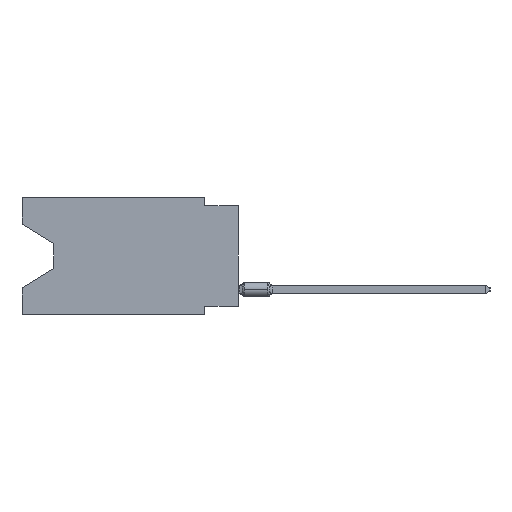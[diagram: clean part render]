
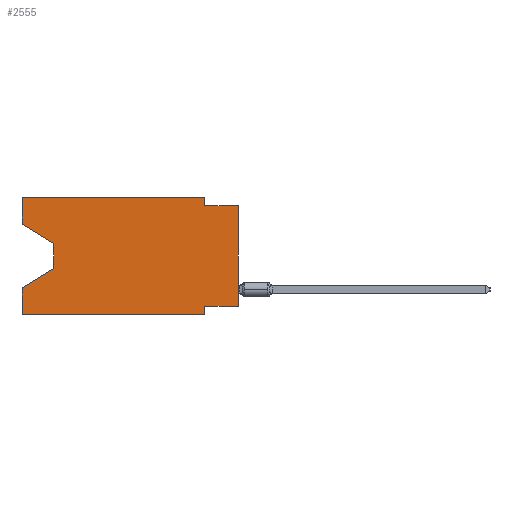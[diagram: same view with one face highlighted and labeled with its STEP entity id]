
A CAD part, left-side view. The second image highlights one B-rep face of the part: STEP entity #2555.
In plain terms, the highlighted planar face has unit normal (-1, 0, 0).
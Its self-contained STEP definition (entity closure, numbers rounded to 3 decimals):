
#773 = CARTESIAN_POINT ( 'NONE',  ( 0., 0., -8.255 ) ) ;
#1943 = VERTEX_POINT ( 'NONE', #59058 ) ;
#2044 = DIRECTION ( 'NONE',  ( 0., 0., 1. ) ) ;
#2555 = ADVANCED_FACE ( 'NONE', ( #10626 ), #63300, .F. ) ;
#4175 = LINE ( 'NONE', #31580, #84136 ) ;
#5321 = ORIENTED_EDGE ( 'NONE', *, *, #13146, .T. ) ;
#7970 = DIRECTION ( 'NONE',  ( 0., -0.855, -0.519 ) ) ;
#10300 = CARTESIAN_POINT ( 'NONE',  ( 0., 16.383, 0. ) ) ;
#10534 = DIRECTION ( 'NONE',  ( 0., 0.855, -0.519 ) ) ;
#10626 = FACE_OUTER_BOUND ( 'NONE', #75087, .T. ) ;
#11880 = CARTESIAN_POINT ( 'NONE',  ( 0., 13.97, -3.505 ) ) ;
#13146 = EDGE_CURVE ( 'NONE', #66226, #49099, #35768, .T. ) ;
#13833 = CARTESIAN_POINT ( 'NONE',  ( 0., 16.383, -8.89 ) ) ;
#14380 = EDGE_CURVE ( 'NONE', #30830, #36060, #46748, .T. ) ;
#14494 = VERTEX_POINT ( 'NONE', #76696 ) ;
#14936 = VECTOR ( 'NONE', #72689, 1000. ) ;
#15894 = VERTEX_POINT ( 'NONE', #85374 ) ;
#16393 = LINE ( 'NONE', #10300, #48743 ) ;
#17652 = DIRECTION ( 'NONE',  ( 0., 0., 1. ) ) ;
#17924 = LINE ( 'NONE', #30573, #37489 ) ;
#18867 = EDGE_CURVE ( 'NONE', #30830, #35750, #4175, .T. ) ;
#20072 = ORIENTED_EDGE ( 'NONE', *, *, #80646, .F. ) ;
#20726 = LINE ( 'NONE', #73825, #41503 ) ;
#22721 = ORIENTED_EDGE ( 'NONE', *, *, #63101, .F. ) ;
#22913 = DIRECTION ( 'NONE',  ( 0., -1., 0. ) ) ;
#23552 = CARTESIAN_POINT ( 'NONE',  ( 0., 0., 0. ) ) ;
#23562 = EDGE_CURVE ( 'NONE', #66226, #15894, #20726, .T. ) ;
#23611 = ORIENTED_EDGE ( 'NONE', *, *, #74810, .F. ) ;
#25434 = CARTESIAN_POINT ( 'NONE',  ( 0., 2.54, -0.635 ) ) ;
#25750 = ORIENTED_EDGE ( 'NONE', *, *, #42365, .T. ) ;
#29750 = VERTEX_POINT ( 'NONE', #25434 ) ;
#29902 = CARTESIAN_POINT ( 'NONE',  ( 0., 16.383, 0. ) ) ;
#30573 = CARTESIAN_POINT ( 'NONE',  ( 0., 13.97, -5.385 ) ) ;
#30668 = DIRECTION ( 'NONE',  ( 1., 0., 0. ) ) ;
#30769 = ORIENTED_EDGE ( 'NONE', *, *, #36256, .T. ) ;
#30830 = VERTEX_POINT ( 'NONE', #56500 ) ;
#30967 = DIRECTION ( 'NONE',  ( 0., 0., 1. ) ) ;
#31580 = CARTESIAN_POINT ( 'NONE',  ( 0., 16.383, 0. ) ) ;
#32949 = ORIENTED_EDGE ( 'NONE', *, *, #71235, .F. ) ;
#33378 = ORIENTED_EDGE ( 'NONE', *, *, #83034, .T. ) ;
#34547 = ORIENTED_EDGE ( 'NONE', *, *, #18867, .F. ) ;
#34891 = ORIENTED_EDGE ( 'NONE', *, *, #14380, .T. ) ;
#35750 = VERTEX_POINT ( 'NONE', #49121 ) ;
#35768 = LINE ( 'NONE', #23552, #41558 ) ;
#36060 = VERTEX_POINT ( 'NONE', #44738 ) ;
#36088 = VECTOR ( 'NONE', #39337, 1000. ) ;
#36256 = EDGE_CURVE ( 'NONE', #36060, #1943, #44963, .T. ) ;
#37489 = VECTOR ( 'NONE', #10534, 1000. ) ;
#37585 = DIRECTION ( 'NONE',  ( 0., 0., -1. ) ) ;
#39020 = LINE ( 'NONE', #58172, #45667 ) ;
#39337 = DIRECTION ( 'NONE',  ( 0., -1., 0. ) ) ;
#41503 = VECTOR ( 'NONE', #61213, 1000. ) ;
#41558 = VECTOR ( 'NONE', #30967, 1000. ) ;
#42365 = EDGE_CURVE ( 'NONE', #1943, #14494, #17924, .T. ) ;
#44738 = CARTESIAN_POINT ( 'NONE',  ( 0., 13.97, -3.505 ) ) ;
#44902 = ORIENTED_EDGE ( 'NONE', *, *, #23562, .F. ) ;
#44963 = LINE ( 'NONE', #11880, #77875 ) ;
#45667 = VECTOR ( 'NONE', #63842, 1000. ) ;
#46292 = CARTESIAN_POINT ( 'NONE',  ( 0., 16.383, -8.89 ) ) ;
#46719 = LINE ( 'NONE', #46292, #36088 ) ;
#46748 = LINE ( 'NONE', #47176, #75093 ) ;
#47176 = CARTESIAN_POINT ( 'NONE',  ( 0., 16.383, -2.038 ) ) ;
#48743 = VECTOR ( 'NONE', #2044, 1000. ) ;
#49099 = VERTEX_POINT ( 'NONE', #56989 ) ;
#49121 = CARTESIAN_POINT ( 'NONE',  ( 0., 16.383, 0. ) ) ;
#50793 = LINE ( 'NONE', #29902, #50795 ) ;
#50795 = VECTOR ( 'NONE', #22913, 1000. ) ;
#54393 = CARTESIAN_POINT ( 'NONE',  ( 0., 2.54, 0. ) ) ;
#55626 = VERTEX_POINT ( 'NONE', #76651 ) ;
#56500 = CARTESIAN_POINT ( 'NONE',  ( 0., 16.383, -2.038 ) ) ;
#56656 = CARTESIAN_POINT ( 'NONE',  ( 0., 2.54, -8.89 ) ) ;
#56989 = CARTESIAN_POINT ( 'NONE',  ( 0., 0., -0.635 ) ) ;
#58171 = DIRECTION ( 'NONE',  ( 0., 0., -1. ) ) ;
#58172 = CARTESIAN_POINT ( 'NONE',  ( 0., 0., -0.635 ) ) ;
#58501 = DIRECTION ( 'NONE',  ( 0., 0., -1. ) ) ;
#59023 = CARTESIAN_POINT ( 'NONE',  ( 0., 2.54, -8.89 ) ) ;
#59058 = CARTESIAN_POINT ( 'NONE',  ( 0., 13.97, -5.385 ) ) ;
#60077 = LINE ( 'NONE', #54393, #14936 ) ;
#61213 = DIRECTION ( 'NONE',  ( 0., 1., 0. ) ) ;
#62980 = EDGE_CURVE ( 'NONE', #35750, #55626, #50793, .T. ) ;
#63101 = EDGE_CURVE ( 'NONE', #15894, #65579, #64697, .T. ) ;
#63300 = PLANE ( 'NONE',  #76368 ) ;
#63842 = DIRECTION ( 'NONE',  ( 0., -1., 0. ) ) ;
#64697 = LINE ( 'NONE', #59023, #75792 ) ;
#65579 = VERTEX_POINT ( 'NONE', #56656 ) ;
#65891 = ORIENTED_EDGE ( 'NONE', *, *, #62980, .F. ) ;
#66137 = VERTEX_POINT ( 'NONE', #13833 ) ;
#66226 = VERTEX_POINT ( 'NONE', #773 ) ;
#71235 = EDGE_CURVE ( 'NONE', #29750, #49099, #39020, .T. ) ;
#72689 = DIRECTION ( 'NONE',  ( 0., 0., -1. ) ) ;
#73825 = CARTESIAN_POINT ( 'NONE',  ( 0., 0., -8.255 ) ) ;
#74810 = EDGE_CURVE ( 'NONE', #66137, #14494, #16393, .T. ) ;
#75087 = EDGE_LOOP ( 'NONE', ( #34891, #30769, #25750, #23611, #33378, #22721, #44902, #5321, #32949, #20072, #65891, #34547 ) ) ;
#75093 = VECTOR ( 'NONE', #7970, 1000. ) ;
#75792 = VECTOR ( 'NONE', #58171, 1000. ) ;
#76368 = AXIS2_PLACEMENT_3D ( 'NONE', #77629, #30668, #58501 ) ;
#76651 = CARTESIAN_POINT ( 'NONE',  ( 0., 2.54, 0. ) ) ;
#76696 = CARTESIAN_POINT ( 'NONE',  ( 0., 16.383, -6.852 ) ) ;
#77629 = CARTESIAN_POINT ( 'NONE',  ( 0., 16.383, 0. ) ) ;
#77875 = VECTOR ( 'NONE', #37585, 1000. ) ;
#80646 = EDGE_CURVE ( 'NONE', #55626, #29750, #60077, .T. ) ;
#83034 = EDGE_CURVE ( 'NONE', #66137, #65579, #46719, .T. ) ;
#84136 = VECTOR ( 'NONE', #17652, 1000. ) ;
#85374 = CARTESIAN_POINT ( 'NONE',  ( 0., 2.54, -8.255 ) ) ;
